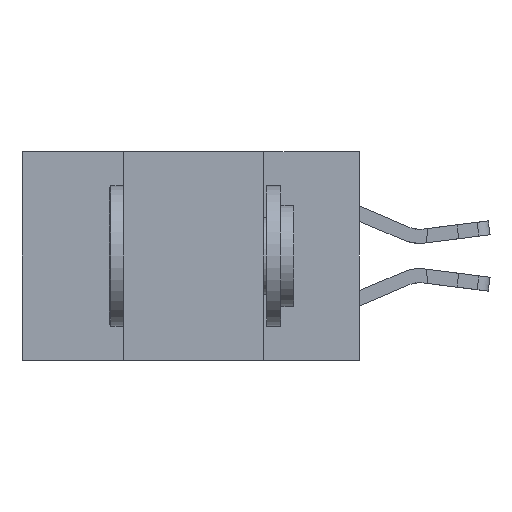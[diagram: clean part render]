
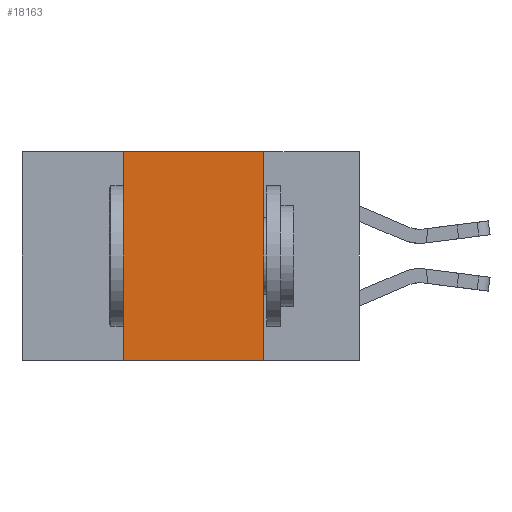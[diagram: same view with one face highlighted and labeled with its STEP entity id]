
A CAD part, left-side view. The second image highlights one B-rep face of the part: STEP entity #18163.
In plain terms, the highlighted planar face has unit normal (-1, 0, 0).
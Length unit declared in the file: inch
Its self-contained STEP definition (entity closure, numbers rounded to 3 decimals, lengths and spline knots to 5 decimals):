
#556 = AXIS2_PLACEMENT_3D ( 'NONE', #8542, #19303, #27397 ) ;
#569 = PLANE ( 'NONE',  #556 ) ;
#1798 = EDGE_CURVE ( 'NONE', #23589, #14527, #20270, .T. ) ;
#1831 = CARTESIAN_POINT ( 'NONE',  ( 0., 0.42, 0. ) ) ;
#3452 = VECTOR ( 'NONE', #25924, 39.37008 ) ;
#6392 = VECTOR ( 'NONE', #33320, 39.37008 ) ;
#6412 = FACE_OUTER_BOUND ( 'NONE', #19346, .T. ) ;
#6560 = DIRECTION ( 'NONE',  ( 0., 0., -1. ) ) ;
#7110 = DIRECTION ( 'NONE',  ( 0., 0., 1. ) ) ;
#8447 = EDGE_CURVE ( 'NONE', #17987, #14527, #27305, .T. ) ;
#8542 = CARTESIAN_POINT ( 'NONE',  ( 0., 0.6, 0. ) ) ;
#14527 = VERTEX_POINT ( 'NONE', #15129 ) ;
#14772 = CARTESIAN_POINT ( 'NONE',  ( 0., 0.17, 0. ) ) ;
#15129 = CARTESIAN_POINT ( 'NONE',  ( 0., 0.17, -0.37 ) ) ;
#17078 = CARTESIAN_POINT ( 'NONE',  ( 0., 0.6, -0.37 ) ) ;
#17687 = CARTESIAN_POINT ( 'NONE',  ( 0., 0.6, 0. ) ) ;
#17987 = VERTEX_POINT ( 'NONE', #28599 ) ;
#18073 = ORIENTED_EDGE ( 'NONE', *, *, #1798, .T. ) ;
#18163 = ADVANCED_FACE ( 'NONE', ( #6412 ), #569, .F. ) ;
#19303 = DIRECTION ( 'NONE',  ( 1., 0., 0. ) ) ;
#19346 = EDGE_LOOP ( 'NONE', ( #32385, #34177, #31439, #18073 ) ) ;
#20270 = LINE ( 'NONE', #17078, #6392 ) ;
#22626 = CARTESIAN_POINT ( 'NONE',  ( 0., 0.42, -0.37 ) ) ;
#23170 = VECTOR ( 'NONE', #6560, 39.37008 ) ;
#23181 = LINE ( 'NONE', #17687, #3452 ) ;
#23589 = VERTEX_POINT ( 'NONE', #22626 ) ;
#25900 = VECTOR ( 'NONE', #7110, 39.37008 ) ;
#25924 = DIRECTION ( 'NONE',  ( 0., -1., 0. ) ) ;
#27305 = LINE ( 'NONE', #14772, #23170 ) ;
#27397 = DIRECTION ( 'NONE',  ( 0., 0., -1. ) ) ;
#27728 = EDGE_CURVE ( 'NONE', #34158, #17987, #23181, .T. ) ;
#28599 = CARTESIAN_POINT ( 'NONE',  ( 0., 0.17, 0. ) ) ;
#30369 = EDGE_CURVE ( 'NONE', #23589, #34158, #33044, .T. ) ;
#30507 = CARTESIAN_POINT ( 'NONE',  ( 0., 0.42, 0. ) ) ;
#31439 = ORIENTED_EDGE ( 'NONE', *, *, #30369, .F. ) ;
#32385 = ORIENTED_EDGE ( 'NONE', *, *, #8447, .F. ) ;
#33044 = LINE ( 'NONE', #1831, #25900 ) ;
#33320 = DIRECTION ( 'NONE',  ( 0., -1., 0. ) ) ;
#34158 = VERTEX_POINT ( 'NONE', #30507 ) ;
#34177 = ORIENTED_EDGE ( 'NONE', *, *, #27728, .F. ) ;
